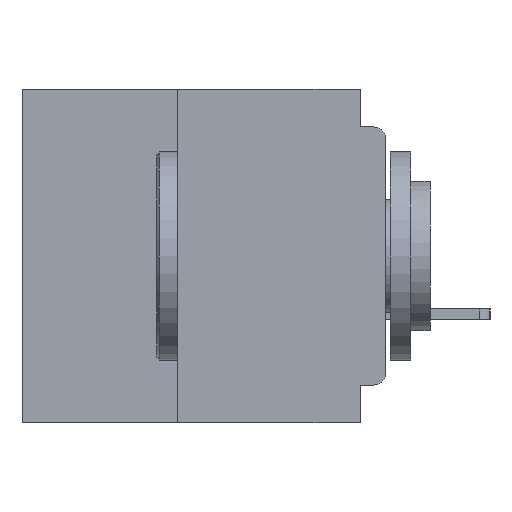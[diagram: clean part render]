
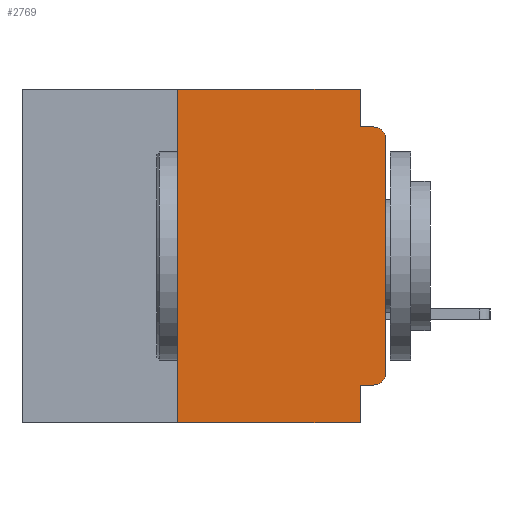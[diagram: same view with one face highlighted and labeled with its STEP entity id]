
A CAD part, left-side view. The second image highlights one B-rep face of the part: STEP entity #2769.
In plain terms, the highlighted planar face has unit normal (-1, 0, 0).
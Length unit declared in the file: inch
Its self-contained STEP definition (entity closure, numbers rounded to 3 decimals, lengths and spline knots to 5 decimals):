
#72 = CARTESIAN_POINT ( 'NONE',  ( 0., 0.031, -0.355 ) ) ;
#2769 = ADVANCED_FACE ( 'NONE', ( #20514 ), #13213, .F. ) ;
#2770 = DIRECTION ( 'NONE',  ( -1., 0., 0. ) ) ;
#2957 = VECTOR ( 'NONE', #42070, 39.37008 ) ;
#3105 = VERTEX_POINT ( 'NONE', #72 ) ;
#3832 = CARTESIAN_POINT ( 'NONE',  ( 0., 0.25, -0.4 ) ) ;
#3964 = EDGE_CURVE ( 'NONE', #21121, #3978, #5191, .T. ) ;
#3978 = VERTEX_POINT ( 'NONE', #21671 ) ;
#4361 = DIRECTION ( 'NONE',  ( 0., -1., 0. ) ) ;
#4631 = DIRECTION ( 'NONE',  ( 0., -1., 0. ) ) ;
#5023 = LINE ( 'NONE', #11777, #43708 ) ;
#5191 = CIRCLE ( 'NONE', #36002, 0.015 ) ;
#5421 = CARTESIAN_POINT ( 'NONE',  ( 0., 0.015, -0.355 ) ) ;
#5426 = ORIENTED_EDGE ( 'NONE', *, *, #19864, .F. ) ;
#5549 = VECTOR ( 'NONE', #4631, 39.37008 ) ;
#6563 = DIRECTION ( 'NONE',  ( 0., -1., 0. ) ) ;
#7580 = VECTOR ( 'NONE', #26783, 39.37008 ) ;
#7656 = DIRECTION ( 'NONE',  ( 0., 0., 1. ) ) ;
#8661 = AXIS2_PLACEMENT_3D ( 'NONE', #12021, #11979, #11916 ) ;
#8731 = LINE ( 'NONE', #45427, #7580 ) ;
#9469 = VECTOR ( 'NONE', #6563, 39.37008 ) ;
#9623 = EDGE_CURVE ( 'NONE', #16411, #43711, #5023, .T. ) ;
#11323 = ORIENTED_EDGE ( 'NONE', *, *, #18225, .F. ) ;
#11777 = CARTESIAN_POINT ( 'NONE',  ( 0., 0., -0.045 ) ) ;
#11916 = DIRECTION ( 'NONE',  ( 0., 0., -1. ) ) ;
#11920 = ORIENTED_EDGE ( 'NONE', *, *, #33835, .F. ) ;
#11979 = DIRECTION ( 'NONE',  ( 1., 0., 0. ) ) ;
#12021 = CARTESIAN_POINT ( 'NONE',  ( 0., 0.437, 0. ) ) ;
#12377 = EDGE_CURVE ( 'NONE', #3105, #29236, #27047, .T. ) ;
#12453 = VERTEX_POINT ( 'NONE', #36631 ) ;
#13213 = PLANE ( 'NONE',  #8661 ) ;
#13385 = CARTESIAN_POINT ( 'NONE',  ( 0., 0.25, 0. ) ) ;
#13646 = VERTEX_POINT ( 'NONE', #31265 ) ;
#14383 = LINE ( 'NONE', #37937, #43104 ) ;
#14910 = ORIENTED_EDGE ( 'NONE', *, *, #33045, .F. ) ;
#15106 = EDGE_CURVE ( 'NONE', #46396, #43711, #43324, .T. ) ;
#15161 = LINE ( 'NONE', #3832, #43871 ) ;
#15518 = ORIENTED_EDGE ( 'NONE', *, *, #3964, .T. ) ;
#15828 = CARTESIAN_POINT ( 'NONE',  ( 0., 0.031, 0. ) ) ;
#16411 = VERTEX_POINT ( 'NONE', #24099 ) ;
#17111 = VECTOR ( 'NONE', #21173, 39.37008 ) ;
#17676 = CARTESIAN_POINT ( 'NONE',  ( 0., 0.437, -0.4 ) ) ;
#17979 = CARTESIAN_POINT ( 'NONE',  ( 0., 0.031, -0.4 ) ) ;
#18225 = EDGE_CURVE ( 'NONE', #35427, #12453, #35466, .T. ) ;
#19864 = EDGE_CURVE ( 'NONE', #12453, #16411, #30518, .T. ) ;
#19984 = ORIENTED_EDGE ( 'NONE', *, *, #15106, .T. ) ;
#20514 = FACE_OUTER_BOUND ( 'NONE', #47800, .T. ) ;
#21121 = VERTEX_POINT ( 'NONE', #5421 ) ;
#21173 = DIRECTION ( 'NONE',  ( 0., 0., -1. ) ) ;
#21671 = CARTESIAN_POINT ( 'NONE',  ( 0., 0., -0.34 ) ) ;
#21869 = AXIS2_PLACEMENT_3D ( 'NONE', #25188, #2770, #28978 ) ;
#22383 = DIRECTION ( 'NONE',  ( 0., 0., -1. ) ) ;
#22548 = DIRECTION ( 'NONE',  ( -1., 0., 0. ) ) ;
#22963 = DIRECTION ( 'NONE',  ( 0., 0., 1. ) ) ;
#22967 = CARTESIAN_POINT ( 'NONE',  ( 0., 0.015, -0.34 ) ) ;
#23052 = ORIENTED_EDGE ( 'NONE', *, *, #25081, .T. ) ;
#24099 = CARTESIAN_POINT ( 'NONE',  ( 0., 0.031, -0.045 ) ) ;
#25081 = EDGE_CURVE ( 'NONE', #13646, #29236, #26961, .T. ) ;
#25188 = CARTESIAN_POINT ( 'NONE',  ( 0., 0.015, -0.06 ) ) ;
#25249 = ORIENTED_EDGE ( 'NONE', *, *, #28189, .T. ) ;
#25476 = CARTESIAN_POINT ( 'NONE',  ( 0., 0., -0.06 ) ) ;
#26783 = DIRECTION ( 'NONE',  ( 0., 1., 0. ) ) ;
#26961 = LINE ( 'NONE', #17676, #9469 ) ;
#27042 = ORIENTED_EDGE ( 'NONE', *, *, #9623, .F. ) ;
#27047 = LINE ( 'NONE', #47314, #17111 ) ;
#28189 = EDGE_CURVE ( 'NONE', #3978, #46396, #14383, .T. ) ;
#28978 = DIRECTION ( 'NONE',  ( 0., 0., -1. ) ) ;
#29236 = VERTEX_POINT ( 'NONE', #17979 ) ;
#30131 = ORIENTED_EDGE ( 'NONE', *, *, #12377, .F. ) ;
#30518 = LINE ( 'NONE', #15828, #2957 ) ;
#31265 = CARTESIAN_POINT ( 'NONE',  ( 0., 0.25, -0.4 ) ) ;
#33045 = EDGE_CURVE ( 'NONE', #21121, #3105, #8731, .T. ) ;
#33835 = EDGE_CURVE ( 'NONE', #13646, #35427, #15161, .T. ) ;
#35427 = VERTEX_POINT ( 'NONE', #13385 ) ;
#35466 = LINE ( 'NONE', #45692, #5549 ) ;
#35731 = CARTESIAN_POINT ( 'NONE',  ( 0., 0.015, -0.045 ) ) ;
#36002 = AXIS2_PLACEMENT_3D ( 'NONE', #22967, #22548, #22383 ) ;
#36631 = CARTESIAN_POINT ( 'NONE',  ( 0., 0.031, 0. ) ) ;
#37937 = CARTESIAN_POINT ( 'NONE',  ( 0., 0., 0. ) ) ;
#42070 = DIRECTION ( 'NONE',  ( 0., 0., -1. ) ) ;
#43104 = VECTOR ( 'NONE', #22963, 39.37008 ) ;
#43324 = CIRCLE ( 'NONE', #21869, 0.015 ) ;
#43708 = VECTOR ( 'NONE', #4361, 39.37008 ) ;
#43711 = VERTEX_POINT ( 'NONE', #35731 ) ;
#43871 = VECTOR ( 'NONE', #7656, 39.37008 ) ;
#45427 = CARTESIAN_POINT ( 'NONE',  ( 0., 0., -0.355 ) ) ;
#45692 = CARTESIAN_POINT ( 'NONE',  ( 0., 0.437, 0. ) ) ;
#46396 = VERTEX_POINT ( 'NONE', #25476 ) ;
#47314 = CARTESIAN_POINT ( 'NONE',  ( 0., 0.031, -0.4 ) ) ;
#47800 = EDGE_LOOP ( 'NONE', ( #25249, #19984, #27042, #5426, #11323, #11920, #23052, #30131, #14910, #15518 ) ) ;
